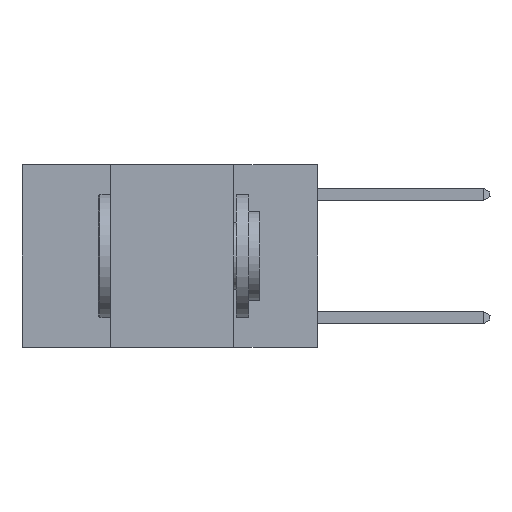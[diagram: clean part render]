
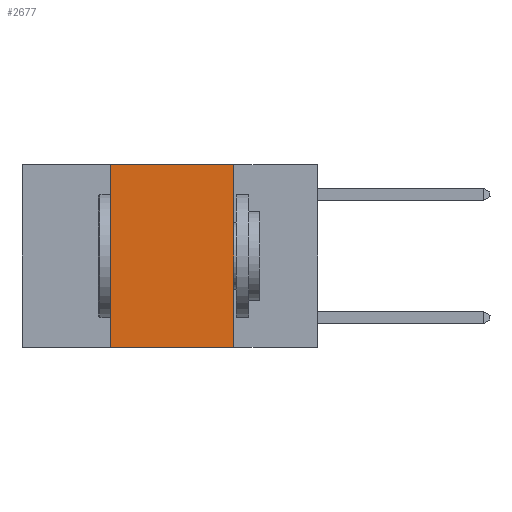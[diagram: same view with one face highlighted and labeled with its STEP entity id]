
A CAD part, left-side view. The second image highlights one B-rep face of the part: STEP entity #2677.
In plain terms, the highlighted planar face has unit normal (-1, 0, 0).
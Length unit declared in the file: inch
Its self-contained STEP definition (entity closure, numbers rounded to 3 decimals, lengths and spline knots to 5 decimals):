
#1465 = DIRECTION ( 'NONE',  ( 0., 0., -1. ) ) ;
#1785 = CARTESIAN_POINT ( 'NONE',  ( 0., 0.6, 0. ) ) ;
#1948 = AXIS2_PLACEMENT_3D ( 'NONE', #1785, #3528, #9119 ) ;
#2167 = LINE ( 'NONE', #19719, #3132 ) ;
#2677 = ADVANCED_FACE ( 'NONE', ( #5500 ), #16312, .F. ) ;
#2849 = LINE ( 'NONE', #7959, #8631 ) ;
#3132 = VECTOR ( 'NONE', #21365, 39.37008 ) ;
#3528 = DIRECTION ( 'NONE',  ( 1., 0., 0. ) ) ;
#3953 = VERTEX_POINT ( 'NONE', #17613 ) ;
#4020 = ORIENTED_EDGE ( 'NONE', *, *, #10943, .F. ) ;
#4490 = ORIENTED_EDGE ( 'NONE', *, *, #11823, .F. ) ;
#4791 = ORIENTED_EDGE ( 'NONE', *, *, #9982, .T. ) ;
#5093 = LINE ( 'NONE', #18948, #10951 ) ;
#5500 = FACE_OUTER_BOUND ( 'NONE', #13575, .T. ) ;
#6216 = DIRECTION ( 'NONE',  ( 0., -1., 0. ) ) ;
#7959 = CARTESIAN_POINT ( 'NONE',  ( 0., 0.6, -0.37 ) ) ;
#8467 = ORIENTED_EDGE ( 'NONE', *, *, #9670, .F. ) ;
#8631 = VECTOR ( 'NONE', #6216, 39.37008 ) ;
#8905 = CARTESIAN_POINT ( 'NONE',  ( 0., 0.17, 0. ) ) ;
#9119 = DIRECTION ( 'NONE',  ( 0., 0., -1. ) ) ;
#9670 = EDGE_CURVE ( 'NONE', #19467, #15122, #14372, .T. ) ;
#9916 = CARTESIAN_POINT ( 'NONE',  ( 0., 0.17, 0. ) ) ;
#9982 = EDGE_CURVE ( 'NONE', #15201, #15122, #2849, .T. ) ;
#10335 = CARTESIAN_POINT ( 'NONE',  ( 0., 0.17, -0.37 ) ) ;
#10943 = EDGE_CURVE ( 'NONE', #15201, #3953, #5093, .T. ) ;
#10951 = VECTOR ( 'NONE', #19278, 39.37008 ) ;
#11823 = EDGE_CURVE ( 'NONE', #3953, #19467, #2167, .T. ) ;
#12633 = CARTESIAN_POINT ( 'NONE',  ( 0., 0.42, -0.37 ) ) ;
#13575 = EDGE_LOOP ( 'NONE', ( #8467, #4490, #4020, #4791 ) ) ;
#13825 = VECTOR ( 'NONE', #1465, 39.37008 ) ;
#14372 = LINE ( 'NONE', #8905, #13825 ) ;
#15122 = VERTEX_POINT ( 'NONE', #10335 ) ;
#15201 = VERTEX_POINT ( 'NONE', #12633 ) ;
#16312 = PLANE ( 'NONE',  #1948 ) ;
#17613 = CARTESIAN_POINT ( 'NONE',  ( 0., 0.42, 0. ) ) ;
#18948 = CARTESIAN_POINT ( 'NONE',  ( 0., 0.42, 0. ) ) ;
#19278 = DIRECTION ( 'NONE',  ( 0., 0., 1. ) ) ;
#19467 = VERTEX_POINT ( 'NONE', #9916 ) ;
#19719 = CARTESIAN_POINT ( 'NONE',  ( 0., 0.6, 0. ) ) ;
#21365 = DIRECTION ( 'NONE',  ( 0., -1., 0. ) ) ;
